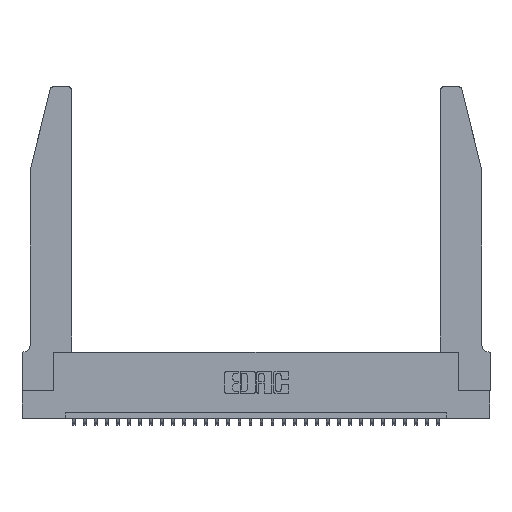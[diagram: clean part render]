
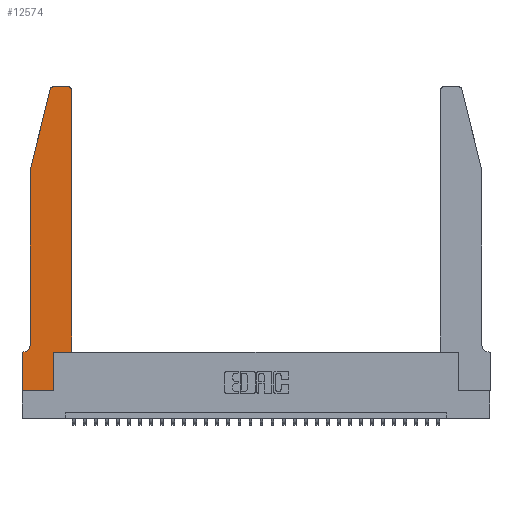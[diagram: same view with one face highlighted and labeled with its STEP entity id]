
A CAD part, top view. The second image highlights one B-rep face of the part: STEP entity #12574.
In plain terms, the highlighted planar face has unit normal (0, 0, 1).
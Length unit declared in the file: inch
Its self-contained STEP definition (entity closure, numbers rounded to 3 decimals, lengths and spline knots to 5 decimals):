
#317 = ORIENTED_EDGE ( 'NONE', *, *, #25589, .T. ) ;
#601 = CARTESIAN_POINT ( 'NONE',  ( 0., 0., 0.37 ) ) ;
#1625 = EDGE_CURVE ( 'NONE', #6693, #29501, #30855, .T. ) ;
#1745 = VECTOR ( 'NONE', #21447, 39.37008 ) ;
#1950 = CARTESIAN_POINT ( 'NONE',  ( 0.0055, 0.42, 0.37 ) ) ;
#2069 = CARTESIAN_POINT ( 'NONE',  ( 0., 0.35, 0.37 ) ) ;
#2113 = CARTESIAN_POINT ( 'NONE',  ( 0.2865, 0.35, 0.37 ) ) ;
#2390 = LINE ( 'NONE', #14068, #21771 ) ;
#2588 = CARTESIAN_POINT ( 'NONE',  ( 0.2865, 0.35, 0.37 ) ) ;
#3223 = CARTESIAN_POINT ( 'NONE',  ( 0.0755, 0.35, 0.37 ) ) ;
#3506 = EDGE_CURVE ( 'NONE', #12224, #22583, #2390, .T. ) ;
#3517 = CARTESIAN_POINT ( 'NONE',  ( 0.4505, 0.35, 0.37 ) ) ;
#3823 = CIRCLE ( 'NONE', #14433, 0.07 ) ;
#4165 = DIRECTION ( 'NONE',  ( 1., 0., 0. ) ) ;
#4259 = CARTESIAN_POINT ( 'NONE',  ( 0.0755, 2., 0.37 ) ) ;
#4379 = ORIENTED_EDGE ( 'NONE', *, *, #30437, .T. ) ;
#4479 = CARTESIAN_POINT ( 'NONE',  ( 0.2605, 2.75, 0.37 ) ) ;
#5723 = LINE ( 'NONE', #4259, #24368 ) ;
#5975 = CARTESIAN_POINT ( 'NONE',  ( 0., 0.35, 0.37 ) ) ;
#6693 = VERTEX_POINT ( 'NONE', #16156 ) ;
#6931 = VERTEX_POINT ( 'NONE', #13329 ) ;
#7059 = ORIENTED_EDGE ( 'NONE', *, *, #27869, .T. ) ;
#8164 = VERTEX_POINT ( 'NONE', #11211 ) ;
#8367 = CARTESIAN_POINT ( 'NONE',  ( 0.284, 2.72, 0.37 ) ) ;
#8954 = VERTEX_POINT ( 'NONE', #30333 ) ;
#9007 = DIRECTION ( 'NONE',  ( 0., 1., 0. ) ) ;
#9388 = LINE ( 'NONE', #3517, #11256 ) ;
#9763 = CARTESIAN_POINT ( 'NONE',  ( 0.2865, 0., 0.37 ) ) ;
#9852 = ORIENTED_EDGE ( 'NONE', *, *, #21612, .T. ) ;
#9864 = LINE ( 'NONE', #21986, #21713 ) ;
#10122 = DIRECTION ( 'NONE',  ( 1., 0., 0. ) ) ;
#10193 = EDGE_CURVE ( 'NONE', #29835, #12224, #9388, .T. ) ;
#10431 = DIRECTION ( 'NONE',  ( -1., 0., 0. ) ) ;
#10720 = CARTESIAN_POINT ( 'NONE',  ( 0., 0., 0.37 ) ) ;
#10745 = ORIENTED_EDGE ( 'NONE', *, *, #30274, .T. ) ;
#11211 = CARTESIAN_POINT ( 'NONE',  ( 0., 0., 0.37 ) ) ;
#11256 = VECTOR ( 'NONE', #20512, 39.37008 ) ;
#12224 = VERTEX_POINT ( 'NONE', #12938 ) ;
#12574 = ADVANCED_FACE ( 'NONE', ( #18738 ), #30989, .T. ) ;
#12938 = CARTESIAN_POINT ( 'NONE',  ( 0.4505, 0.35, 0.37 ) ) ;
#13023 = DIRECTION ( 'NONE',  ( 1., 0., 0. ) ) ;
#13329 = CARTESIAN_POINT ( 'NONE',  ( 0.25487, 2.72718, 0.37 ) ) ;
#14068 = CARTESIAN_POINT ( 'NONE',  ( 0.4505, 0.35, 0.37 ) ) ;
#14412 = ORIENTED_EDGE ( 'NONE', *, *, #10193, .T. ) ;
#14433 = AXIS2_PLACEMENT_3D ( 'NONE', #1950, #21489, #31405 ) ;
#14474 = EDGE_CURVE ( 'NONE', #29501, #6931, #16401, .T. ) ;
#14531 = AXIS2_PLACEMENT_3D ( 'NONE', #2069, #21403, #4165 ) ;
#14660 = EDGE_CURVE ( 'NONE', #8164, #20187, #25845, .T. ) ;
#14878 = DIRECTION ( 'NONE',  ( 0., 0., 1. ) ) ;
#15763 = VERTEX_POINT ( 'NONE', #5975 ) ;
#16156 = CARTESIAN_POINT ( 'NONE',  ( 0.4205, 2.75, 0.37 ) ) ;
#16397 = ORIENTED_EDGE ( 'NONE', *, *, #24577, .T. ) ;
#16401 = CIRCLE ( 'NONE', #19762, 0.03 ) ;
#16532 = DIRECTION ( 'NONE',  ( -1., 0., 0. ) ) ;
#16553 = ORIENTED_EDGE ( 'NONE', *, *, #14474, .T. ) ;
#17020 = DIRECTION ( 'NONE',  ( 1., 0., 0. ) ) ;
#17208 = ORIENTED_EDGE ( 'NONE', *, *, #26179, .T. ) ;
#18738 = FACE_OUTER_BOUND ( 'NONE', #19194, .T. ) ;
#19194 = EDGE_LOOP ( 'NONE', ( #21693, #16553, #16397, #4379, #10745, #317, #9852, #27706, #7059, #14412, #21697, #17208 ) ) ;
#19762 = AXIS2_PLACEMENT_3D ( 'NONE', #8367, #24020, #17020 ) ;
#20187 = VERTEX_POINT ( 'NONE', #9763 ) ;
#20512 = DIRECTION ( 'NONE',  ( 1., 0., 0. ) ) ;
#20581 = AXIS2_PLACEMENT_3D ( 'NONE', #29405, #14878, #13023 ) ;
#20814 = VECTOR ( 'NONE', #10431, 39.37008 ) ;
#21403 = DIRECTION ( 'NONE',  ( 0., 0., 1. ) ) ;
#21447 = DIRECTION ( 'NONE',  ( 0., 1., 0. ) ) ;
#21489 = DIRECTION ( 'NONE',  ( 0., 0., -1. ) ) ;
#21612 = EDGE_CURVE ( 'NONE', #15763, #8164, #30844, .T. ) ;
#21622 = CIRCLE ( 'NONE', #20581, 0.03 ) ;
#21693 = ORIENTED_EDGE ( 'NONE', *, *, #1625, .T. ) ;
#21697 = ORIENTED_EDGE ( 'NONE', *, *, #3506, .T. ) ;
#21713 = VECTOR ( 'NONE', #22082, 39.37008 ) ;
#21771 = VECTOR ( 'NONE', #9007, 39.37008 ) ;
#21986 = CARTESIAN_POINT ( 'NONE',  ( 0.0755, 2., 0.37 ) ) ;
#22082 = DIRECTION ( 'NONE',  ( 0., -1., 0. ) ) ;
#22583 = VERTEX_POINT ( 'NONE', #24522 ) ;
#22851 = CARTESIAN_POINT ( 'NONE',  ( 0.0055, 0.35, 0.37 ) ) ;
#24020 = DIRECTION ( 'NONE',  ( 0., 0., 1. ) ) ;
#24032 = DIRECTION ( 'NONE',  ( -0.239, -0.971, 0. ) ) ;
#24368 = VECTOR ( 'NONE', #24032, 39.37008 ) ;
#24418 = VERTEX_POINT ( 'NONE', #22851 ) ;
#24522 = CARTESIAN_POINT ( 'NONE',  ( 0.4505, 2.72, 0.37 ) ) ;
#24577 = EDGE_CURVE ( 'NONE', #6931, #29438, #5723, .T. ) ;
#24722 = VECTOR ( 'NONE', #25117, 39.37008 ) ;
#24912 = CARTESIAN_POINT ( 'NONE',  ( 0.284, 2.75, 0.37 ) ) ;
#25019 = CARTESIAN_POINT ( 'NONE',  ( 0.0755, 2., 0.37 ) ) ;
#25103 = VECTOR ( 'NONE', #16532, 39.37008 ) ;
#25117 = DIRECTION ( 'NONE',  ( 0., -1., 0. ) ) ;
#25589 = EDGE_CURVE ( 'NONE', #24418, #15763, #27625, .T. ) ;
#25845 = LINE ( 'NONE', #601, #28103 ) ;
#26179 = EDGE_CURVE ( 'NONE', #22583, #6693, #21622, .T. ) ;
#27625 = LINE ( 'NONE', #3223, #20814 ) ;
#27706 = ORIENTED_EDGE ( 'NONE', *, *, #14660, .T. ) ;
#27869 = EDGE_CURVE ( 'NONE', #20187, #29835, #31044, .T. ) ;
#28103 = VECTOR ( 'NONE', #10122, 39.37008 ) ;
#29405 = CARTESIAN_POINT ( 'NONE',  ( 0.4205, 2.72, 0.37 ) ) ;
#29438 = VERTEX_POINT ( 'NONE', #25019 ) ;
#29501 = VERTEX_POINT ( 'NONE', #24912 ) ;
#29835 = VERTEX_POINT ( 'NONE', #2588 ) ;
#30274 = EDGE_CURVE ( 'NONE', #8954, #24418, #3823, .T. ) ;
#30333 = CARTESIAN_POINT ( 'NONE',  ( 0.0755, 0.42, 0.37 ) ) ;
#30437 = EDGE_CURVE ( 'NONE', #29438, #8954, #9864, .T. ) ;
#30844 = LINE ( 'NONE', #10720, #24722 ) ;
#30855 = LINE ( 'NONE', #4479, #25103 ) ;
#30989 = PLANE ( 'NONE',  #14531 ) ;
#31044 = LINE ( 'NONE', #2113, #1745 ) ;
#31405 = DIRECTION ( 'NONE',  ( -1., 0., 0. ) ) ;
